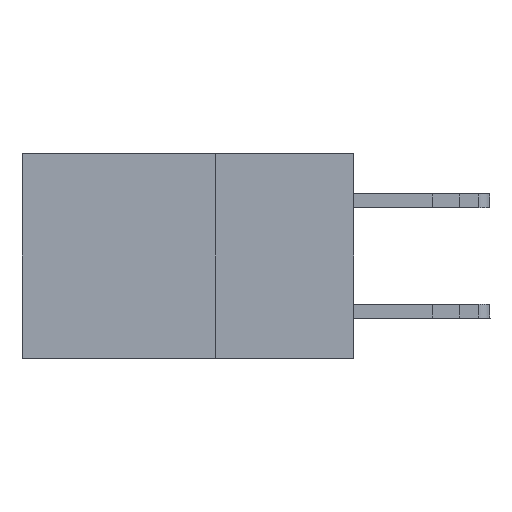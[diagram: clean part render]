
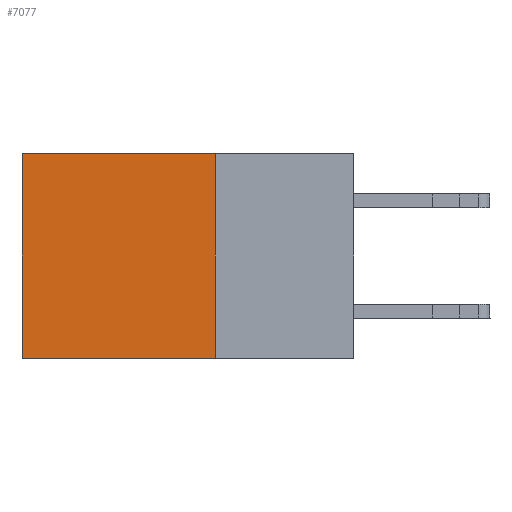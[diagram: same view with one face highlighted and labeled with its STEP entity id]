
A CAD part, left-side view. The second image highlights one B-rep face of the part: STEP entity #7077.
In plain terms, the highlighted planar face has unit normal (-1, 0, 0).
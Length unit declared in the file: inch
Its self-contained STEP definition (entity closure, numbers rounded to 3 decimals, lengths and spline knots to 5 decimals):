
#111 = FACE_OUTER_BOUND ( 'NONE', #1285, .T. ) ;
#406 = VECTOR ( 'NONE', #21493, 39.37008 ) ;
#895 = DIRECTION ( 'NONE',  ( 0., 0., -1. ) ) ;
#967 = LINE ( 'NONE', #5807, #406 ) ;
#1285 = EDGE_LOOP ( 'NONE', ( #15767, #5926, #6450, #7598 ) ) ;
#1449 = CARTESIAN_POINT ( 'NONE',  ( 0.2875, 0.6, 0. ) ) ;
#1972 = LINE ( 'NONE', #19081, #15613 ) ;
#5267 = AXIS2_PLACEMENT_3D ( 'NONE', #20401, #6363, #895 ) ;
#5743 = VERTEX_POINT ( 'NONE', #13030 ) ;
#5807 = CARTESIAN_POINT ( 'NONE',  ( 0.2875, 0.6, 0. ) ) ;
#5836 = VECTOR ( 'NONE', #12862, 39.37008 ) ;
#5926 = ORIENTED_EDGE ( 'NONE', *, *, #15078, .F. ) ;
#6363 = DIRECTION ( 'NONE',  ( 1., 0., 0. ) ) ;
#6450 = ORIENTED_EDGE ( 'NONE', *, *, #12322, .F. ) ;
#6802 = DIRECTION ( 'NONE',  ( 0., 1., 0. ) ) ;
#7077 = ADVANCED_FACE ( 'NONE', ( #111 ), #22084, .F. ) ;
#7598 = ORIENTED_EDGE ( 'NONE', *, *, #13221, .T. ) ;
#8836 = VECTOR ( 'NONE', #19102, 39.37008 ) ;
#10445 = LINE ( 'NONE', #21605, #5836 ) ;
#11954 = CARTESIAN_POINT ( 'NONE',  ( 0.2875, 0.25, 0. ) ) ;
#12322 = EDGE_CURVE ( 'NONE', #13204, #19190, #10445, .T. ) ;
#12862 = DIRECTION ( 'NONE',  ( 0., 0., -1. ) ) ;
#13030 = CARTESIAN_POINT ( 'NONE',  ( 0.2875, 0.6, -0.37 ) ) ;
#13204 = VERTEX_POINT ( 'NONE', #11954 ) ;
#13221 = EDGE_CURVE ( 'NONE', #13204, #17118, #18144, .T. ) ;
#15078 = EDGE_CURVE ( 'NONE', #19190, #5743, #1972, .T. ) ;
#15613 = VECTOR ( 'NONE', #6802, 39.37008 ) ;
#15767 = ORIENTED_EDGE ( 'NONE', *, *, #19235, .T. ) ;
#17118 = VERTEX_POINT ( 'NONE', #1449 ) ;
#17229 = CARTESIAN_POINT ( 'NONE',  ( 0.2875, 0.25, 0. ) ) ;
#18008 = CARTESIAN_POINT ( 'NONE',  ( 0.2875, 0.25, -0.37 ) ) ;
#18144 = LINE ( 'NONE', #17229, #8836 ) ;
#19081 = CARTESIAN_POINT ( 'NONE',  ( 0.2875, 0.25, -0.37 ) ) ;
#19102 = DIRECTION ( 'NONE',  ( 0., 1., 0. ) ) ;
#19190 = VERTEX_POINT ( 'NONE', #18008 ) ;
#19235 = EDGE_CURVE ( 'NONE', #17118, #5743, #967, .T. ) ;
#20401 = CARTESIAN_POINT ( 'NONE',  ( 0.2875, 0.25, 0. ) ) ;
#21493 = DIRECTION ( 'NONE',  ( 0., 0., -1. ) ) ;
#21605 = CARTESIAN_POINT ( 'NONE',  ( 0.2875, 0.25, 0. ) ) ;
#22084 = PLANE ( 'NONE',  #5267 ) ;
